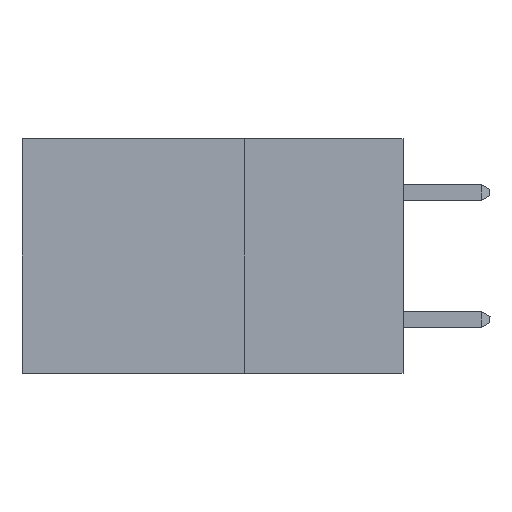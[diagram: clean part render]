
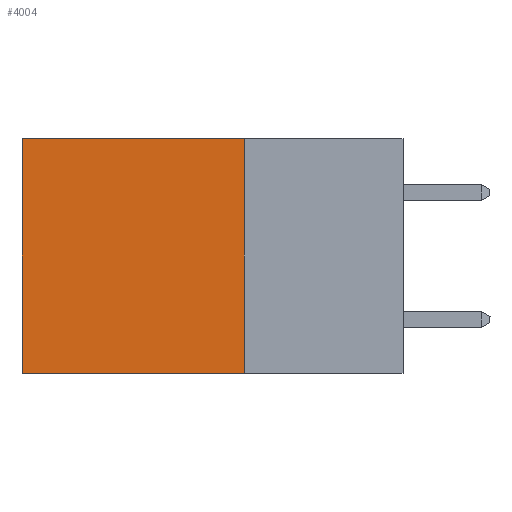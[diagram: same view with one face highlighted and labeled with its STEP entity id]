
A CAD part, left-side view. The second image highlights one B-rep face of the part: STEP entity #4004.
In plain terms, the highlighted planar face has unit normal (-1, 0, 0).
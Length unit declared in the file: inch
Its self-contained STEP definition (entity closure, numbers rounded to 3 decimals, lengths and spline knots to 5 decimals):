
#530 = DIRECTION ( 'NONE',  ( 0., 0., -1. ) ) ;
#549 = VECTOR ( 'NONE', #4971, 39.37008 ) ;
#931 = LINE ( 'NONE', #14354, #549 ) ;
#1008 = VERTEX_POINT ( 'NONE', #8092 ) ;
#1444 = EDGE_LOOP ( 'NONE', ( #16708, #4387, #16011, #7083 ) ) ;
#1451 = CARTESIAN_POINT ( 'NONE',  ( 0.2875, 0.6, 0. ) ) ;
#1508 = LINE ( 'NONE', #14117, #16317 ) ;
#2046 = CARTESIAN_POINT ( 'NONE',  ( 0.2875, 0.6, -0.37 ) ) ;
#3051 = EDGE_CURVE ( 'NONE', #13103, #6791, #9396, .T. ) ;
#4004 = ADVANCED_FACE ( 'NONE', ( #11070 ), #13766, .F. ) ;
#4387 = ORIENTED_EDGE ( 'NONE', *, *, #17080, .F. ) ;
#4971 = DIRECTION ( 'NONE',  ( 0., 1., 0. ) ) ;
#5004 = CARTESIAN_POINT ( 'NONE',  ( 0.2875, 0.25, 0. ) ) ;
#5477 = DIRECTION ( 'NONE',  ( 0., 0., -1. ) ) ;
#6791 = VERTEX_POINT ( 'NONE', #2046 ) ;
#7083 = ORIENTED_EDGE ( 'NONE', *, *, #13338, .T. ) ;
#7101 = DIRECTION ( 'NONE',  ( 0., 1., 0. ) ) ;
#7596 = CARTESIAN_POINT ( 'NONE',  ( 0.2875, 0.25, 0. ) ) ;
#8092 = CARTESIAN_POINT ( 'NONE',  ( 0.2875, 0.25, -0.37 ) ) ;
#8872 = AXIS2_PLACEMENT_3D ( 'NONE', #9507, #9707, #5477 ) ;
#9396 = LINE ( 'NONE', #14984, #10860 ) ;
#9413 = VERTEX_POINT ( 'NONE', #7596 ) ;
#9507 = CARTESIAN_POINT ( 'NONE',  ( 0.2875, 0.25, 0. ) ) ;
#9707 = DIRECTION ( 'NONE',  ( 1., 0., 0. ) ) ;
#10860 = VECTOR ( 'NONE', #17720, 39.37008 ) ;
#11070 = FACE_OUTER_BOUND ( 'NONE', #1444, .T. ) ;
#11436 = VECTOR ( 'NONE', #530, 39.37008 ) ;
#11519 = LINE ( 'NONE', #5004, #11436 ) ;
#13103 = VERTEX_POINT ( 'NONE', #1451 ) ;
#13338 = EDGE_CURVE ( 'NONE', #9413, #13103, #1508, .T. ) ;
#13550 = EDGE_CURVE ( 'NONE', #9413, #1008, #11519, .T. ) ;
#13766 = PLANE ( 'NONE',  #8872 ) ;
#14117 = CARTESIAN_POINT ( 'NONE',  ( 0.2875, 0.25, 0. ) ) ;
#14354 = CARTESIAN_POINT ( 'NONE',  ( 0.2875, 0.25, -0.37 ) ) ;
#14984 = CARTESIAN_POINT ( 'NONE',  ( 0.2875, 0.6, 0. ) ) ;
#16011 = ORIENTED_EDGE ( 'NONE', *, *, #13550, .F. ) ;
#16317 = VECTOR ( 'NONE', #7101, 39.37008 ) ;
#16708 = ORIENTED_EDGE ( 'NONE', *, *, #3051, .T. ) ;
#17080 = EDGE_CURVE ( 'NONE', #1008, #6791, #931, .T. ) ;
#17720 = DIRECTION ( 'NONE',  ( 0., 0., -1. ) ) ;
